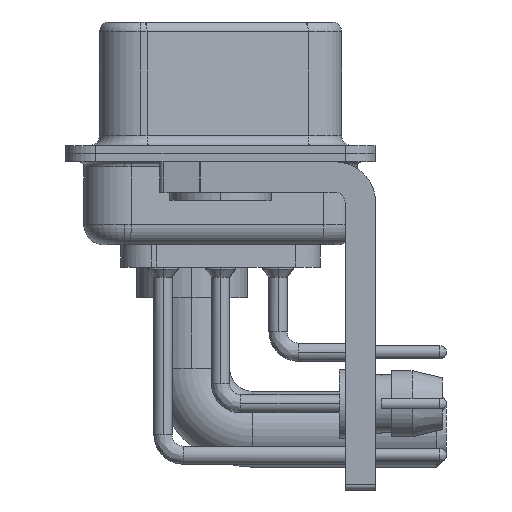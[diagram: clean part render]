
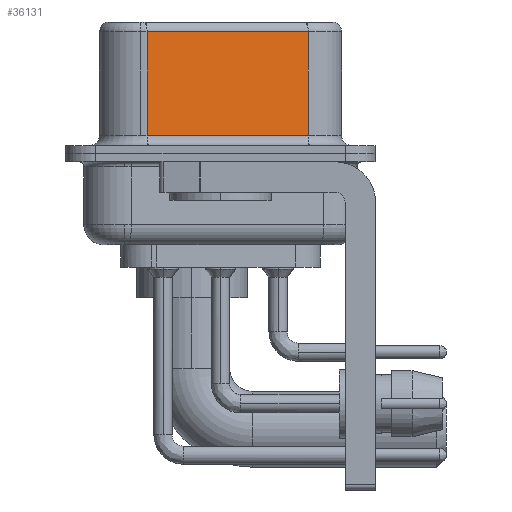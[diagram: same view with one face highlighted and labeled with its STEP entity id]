
A CAD part, left-side view. The second image highlights one B-rep face of the part: STEP entity #36131.
In plain terms, the highlighted planar face has unit normal (-0.985, -0.174, 0).
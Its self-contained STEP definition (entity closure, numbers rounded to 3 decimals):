
#199 = VERTEX_POINT ( 'NONE', #11991 ) ;
#1091 = DIRECTION ( 'NONE',  ( -0.174, 0.985, 0. ) ) ;
#2018 = FACE_OUTER_BOUND ( 'NONE', #11116, .T. ) ;
#2202 = DIRECTION ( 'NONE',  ( -0.174, 0.985, 0. ) ) ;
#2892 = VECTOR ( 'NONE', #23019, 1000. ) ;
#3129 = CARTESIAN_POINT ( 'NONE',  ( 5.132, -4.322, 0.9 ) ) ;
#3650 = LINE ( 'NONE', #21638, #33515 ) ;
#4035 = VERTEX_POINT ( 'NONE', #8973 ) ;
#5522 = AXIS2_PLACEMENT_3D ( 'NONE', #17063, #28975, #2202 ) ;
#5863 = VECTOR ( 'NONE', #1091, 1000. ) ;
#6462 = ORIENTED_EDGE ( 'NONE', *, *, #13309, .T. ) ;
#7606 = CARTESIAN_POINT ( 'NONE',  ( 5.132, -4.322, 0.9 ) ) ;
#7633 = CARTESIAN_POINT ( 'NONE',  ( 3.73, 3.628, 6.52 ) ) ;
#8329 = EDGE_CURVE ( 'NONE', #8600, #12925, #3650, .T. ) ;
#8600 = VERTEX_POINT ( 'NONE', #22038 ) ;
#8973 = CARTESIAN_POINT ( 'NONE',  ( 3.73, 3.628, 0.9 ) ) ;
#10378 = LINE ( 'NONE', #7633, #23049 ) ;
#11116 = EDGE_LOOP ( 'NONE', ( #22803, #23735, #6462, #25294 ) ) ;
#11991 = CARTESIAN_POINT ( 'NONE',  ( 3.73, 3.628, 6.02 ) ) ;
#12453 = DIRECTION ( 'NONE',  ( 0., 0., -1. ) ) ;
#12925 = VERTEX_POINT ( 'NONE', #3129 ) ;
#13309 = EDGE_CURVE ( 'NONE', #199, #4035, #10378, .T. ) ;
#16427 = DIRECTION ( 'NONE',  ( 0., 0., -1. ) ) ;
#17063 = CARTESIAN_POINT ( 'NONE',  ( 5.132, -4.322, 6.52 ) ) ;
#18761 = EDGE_CURVE ( 'NONE', #8600, #199, #28048, .T. ) ;
#21638 = CARTESIAN_POINT ( 'NONE',  ( 5.132, -4.322, 6.52 ) ) ;
#22038 = CARTESIAN_POINT ( 'NONE',  ( 5.132, -4.322, 6.02 ) ) ;
#22803 = ORIENTED_EDGE ( 'NONE', *, *, #8329, .F. ) ;
#23019 = DIRECTION ( 'NONE',  ( 0.174, -0.985, 0. ) ) ;
#23049 = VECTOR ( 'NONE', #16427, 1000. ) ;
#23735 = ORIENTED_EDGE ( 'NONE', *, *, #18761, .T. ) ;
#25294 = ORIENTED_EDGE ( 'NONE', *, *, #30983, .T. ) ;
#25571 = LINE ( 'NONE', #7606, #2892 ) ;
#25657 = PLANE ( 'NONE',  #5522 ) ;
#28048 = LINE ( 'NONE', #30402, #5863 ) ;
#28975 = DIRECTION ( 'NONE',  ( 0.985, 0.174, 0. ) ) ;
#30402 = CARTESIAN_POINT ( 'NONE',  ( 5.132, -4.322, 6.02 ) ) ;
#30983 = EDGE_CURVE ( 'NONE', #4035, #12925, #25571, .T. ) ;
#33515 = VECTOR ( 'NONE', #12453, 1000. ) ;
#36131 = ADVANCED_FACE ( 'NONE', ( #2018 ), #25657, .F. ) ;
